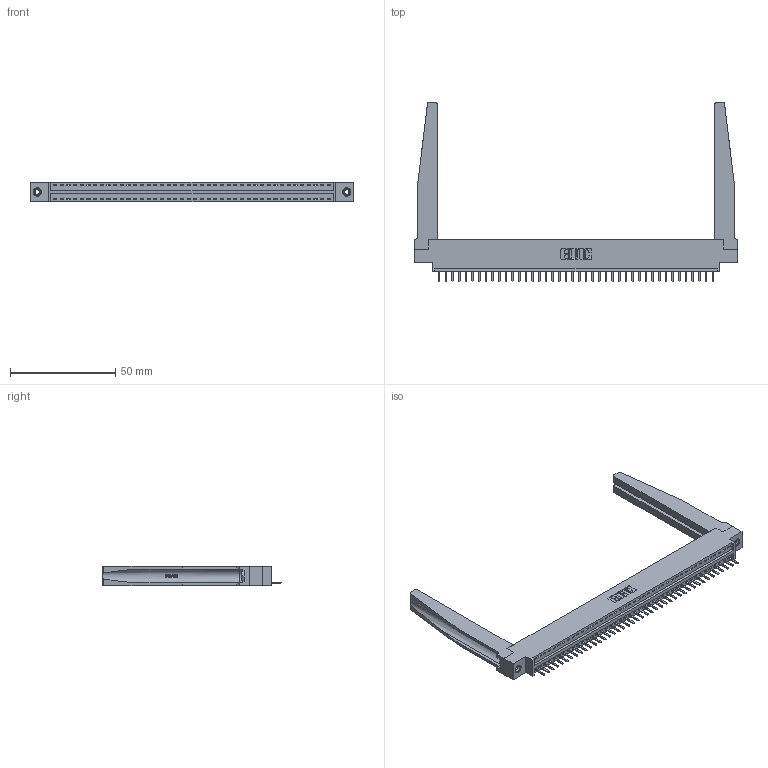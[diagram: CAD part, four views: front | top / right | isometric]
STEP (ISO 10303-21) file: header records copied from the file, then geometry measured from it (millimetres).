
FILE_DESCRIPTION (( 'STEP AP203' ), '1' );
FILE_NAME ('396-042-520-678.STEP', '2019-10-27T21:29:31', ( '' ), ( '' ), 'SwSTEP 2.0', 'SolidWorks 2016', '' );
FILE_SCHEMA (( 'CONFIG_CONTROL_DESIGN' ));
Length unit declared in the file: inch
Products named in the file (5): 346 Part_0.170 Offset - 0.156 Dia-TH; 345-250-001_345-250-001-102; 345-292-001_345-293-120; 396-042-520-678; 346-220-078_345-220-078
Assembly tree (47 placements, depth 2):
  396-042-520-678
    346 Part_0.170 Offset - 0.156 Dia-TH
    345-292-001_345-293-120  x42
    346-220-078_345-220-078  x2
    345-250-001_345-250-001-102  x2
Bounding box: 153.92 x 85.29 x 9.4 mm (x, y, z)
Volume: 21367.4 mm3; surface area: 24368.4 mm2
Topology: 47 solids, 47 shells, 2964 faces, 8677 edges, 5662 vertices
Faces by surface type: plane 1986, cylinder 926, bspline 36, cone 12, torus 4
Entity records: 31060 total; most frequent: CARTESIAN_POINT 6249, ORIENTED_EDGE 5102, DIRECTION 4485, EDGE_CURVE 2551, LINE 2153, VECTOR 2153, VERTEX_POINT 1692, AXIS2_PLACEMENT_3D 1166
